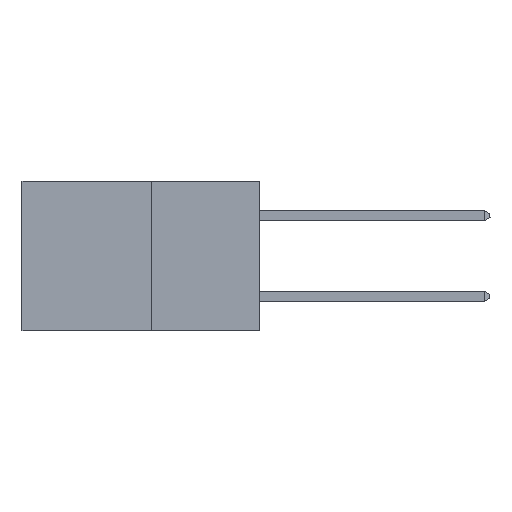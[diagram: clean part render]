
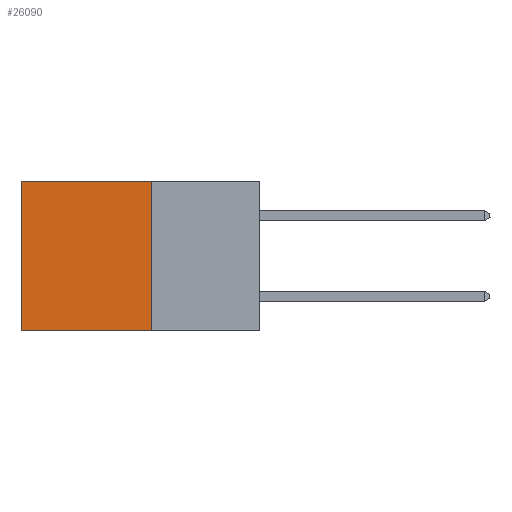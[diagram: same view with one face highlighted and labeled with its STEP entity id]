
A CAD part, left-side view. The second image highlights one B-rep face of the part: STEP entity #26090.
In plain terms, the highlighted planar face has unit normal (-1, 0, 0).
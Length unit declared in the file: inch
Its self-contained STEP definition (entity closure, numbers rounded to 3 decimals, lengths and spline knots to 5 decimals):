
#448 = DIRECTION ( 'NONE',  ( 0., 0., -1. ) ) ;
#455 = CARTESIAN_POINT ( 'NONE',  ( 0.277, 0.27, 0. ) ) ;
#1194 = VECTOR ( 'NONE', #17452, 39.37008 ) ;
#1861 = EDGE_CURVE ( 'NONE', #32089, #13748, #23603, .T. ) ;
#3868 = VECTOR ( 'NONE', #5611, 39.37008 ) ;
#4292 = FACE_OUTER_BOUND ( 'NONE', #17159, .T. ) ;
#4752 = CARTESIAN_POINT ( 'NONE',  ( 0.277, 0.27, -0.37 ) ) ;
#4774 = PLANE ( 'NONE',  #24000 ) ;
#5601 = CARTESIAN_POINT ( 'NONE',  ( 0.277, 0.27, -0.37 ) ) ;
#5611 = DIRECTION ( 'NONE',  ( 0., 1., 0. ) ) ;
#6417 = DIRECTION ( 'NONE',  ( 0., 1., 0. ) ) ;
#7337 = CARTESIAN_POINT ( 'NONE',  ( 0.277, 0.59, -0.37 ) ) ;
#7555 = EDGE_CURVE ( 'NONE', #18422, #26348, #24067, .T. ) ;
#8705 = EDGE_CURVE ( 'NONE', #26348, #13748, #21432, .T. ) ;
#8935 = CARTESIAN_POINT ( 'NONE',  ( 0.277, 0.27, -0.37 ) ) ;
#12323 = EDGE_CURVE ( 'NONE', #18422, #32089, #19547, .T. ) ;
#12399 = DIRECTION ( 'NONE',  ( 1., 0., 0. ) ) ;
#12847 = VECTOR ( 'NONE', #448, 39.37008 ) ;
#13408 = ORIENTED_EDGE ( 'NONE', *, *, #1861, .F. ) ;
#13748 = VERTEX_POINT ( 'NONE', #23419 ) ;
#15784 = CARTESIAN_POINT ( 'NONE',  ( 0.277, 0.59, 0. ) ) ;
#16810 = VECTOR ( 'NONE', #6417, 39.37008 ) ;
#17159 = EDGE_LOOP ( 'NONE', ( #27838, #13408, #18151, #20503 ) ) ;
#17452 = DIRECTION ( 'NONE',  ( 0., 0., -1. ) ) ;
#18151 = ORIENTED_EDGE ( 'NONE', *, *, #12323, .F. ) ;
#18422 = VERTEX_POINT ( 'NONE', #31620 ) ;
#19547 = LINE ( 'NONE', #5601, #12847 ) ;
#20503 = ORIENTED_EDGE ( 'NONE', *, *, #7555, .T. ) ;
#21432 = LINE ( 'NONE', #7337, #1194 ) ;
#23419 = CARTESIAN_POINT ( 'NONE',  ( 0.277, 0.59, -0.37 ) ) ;
#23603 = LINE ( 'NONE', #8935, #16810 ) ;
#24000 = AXIS2_PLACEMENT_3D ( 'NONE', #27531, #12399, #30053 ) ;
#24067 = LINE ( 'NONE', #455, #3868 ) ;
#26090 = ADVANCED_FACE ( 'NONE', ( #4292 ), #4774, .F. ) ;
#26348 = VERTEX_POINT ( 'NONE', #15784 ) ;
#27531 = CARTESIAN_POINT ( 'NONE',  ( 0.277, 0.27, -0.37 ) ) ;
#27838 = ORIENTED_EDGE ( 'NONE', *, *, #8705, .T. ) ;
#30053 = DIRECTION ( 'NONE',  ( 0., 0., -1. ) ) ;
#31620 = CARTESIAN_POINT ( 'NONE',  ( 0.277, 0.27, 0. ) ) ;
#32089 = VERTEX_POINT ( 'NONE', #4752 ) ;
